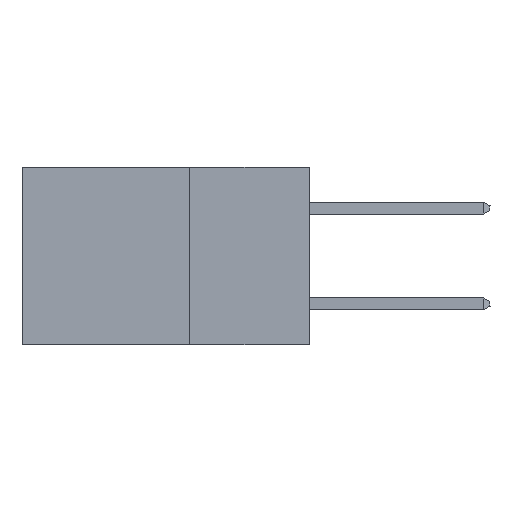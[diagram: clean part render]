
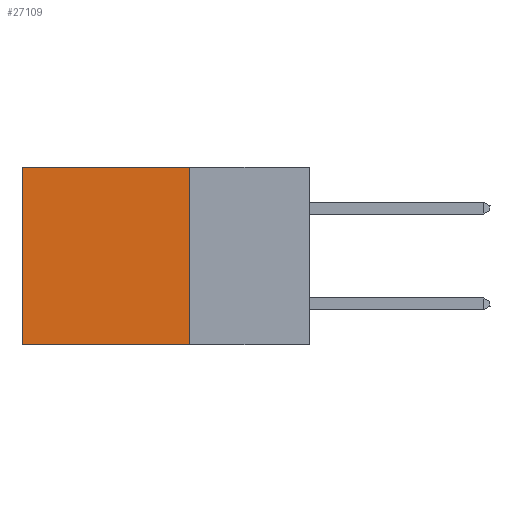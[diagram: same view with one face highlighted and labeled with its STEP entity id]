
A CAD part, left-side view. The second image highlights one B-rep face of the part: STEP entity #27109.
In plain terms, the highlighted planar face has unit normal (-1, 0, 0).
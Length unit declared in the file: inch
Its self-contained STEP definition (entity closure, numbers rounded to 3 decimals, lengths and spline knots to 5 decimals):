
#1278 = LINE ( 'NONE', #23569, #31314 ) ;
#2040 = ORIENTED_EDGE ( 'NONE', *, *, #3856, .F. ) ;
#3856 = EDGE_CURVE ( 'NONE', #38077, #13913, #1278, .T. ) ;
#4476 = ORIENTED_EDGE ( 'NONE', *, *, #10591, .F. ) ;
#5606 = ORIENTED_EDGE ( 'NONE', *, *, #35318, .T. ) ;
#9138 = VERTEX_POINT ( 'NONE', #19583 ) ;
#10522 = DIRECTION ( 'NONE',  ( 0., 0., -1. ) ) ;
#10548 = VECTOR ( 'NONE', #14507, 39.37008 ) ;
#10591 = EDGE_CURVE ( 'NONE', #13913, #19894, #17721, .T. ) ;
#12352 = AXIS2_PLACEMENT_3D ( 'NONE', #17239, #23555, #13992 ) ;
#13142 = CARTESIAN_POINT ( 'NONE',  ( 0.2875, 0.25, 0. ) ) ;
#13913 = VERTEX_POINT ( 'NONE', #36959 ) ;
#13992 = DIRECTION ( 'NONE',  ( 0., 0., -1. ) ) ;
#14507 = DIRECTION ( 'NONE',  ( 0., 1., 0. ) ) ;
#14520 = CARTESIAN_POINT ( 'NONE',  ( 0.2875, 0.6, 0. ) ) ;
#14729 = FACE_OUTER_BOUND ( 'NONE', #18526, .T. ) ;
#15652 = ORIENTED_EDGE ( 'NONE', *, *, #29291, .T. ) ;
#17239 = CARTESIAN_POINT ( 'NONE',  ( 0.2875, 0.25, 0. ) ) ;
#17721 = LINE ( 'NONE', #36675, #35751 ) ;
#18208 = LINE ( 'NONE', #14520, #34228 ) ;
#18526 = EDGE_LOOP ( 'NONE', ( #15652, #4476, #2040, #5606 ) ) ;
#19583 = CARTESIAN_POINT ( 'NONE',  ( 0.2875, 0.6, 0. ) ) ;
#19894 = VERTEX_POINT ( 'NONE', #22205 ) ;
#22205 = CARTESIAN_POINT ( 'NONE',  ( 0.2875, 0.6, -0.37 ) ) ;
#23555 = DIRECTION ( 'NONE',  ( 1., 0., 0. ) ) ;
#23569 = CARTESIAN_POINT ( 'NONE',  ( 0.2875, 0.25, 0. ) ) ;
#27109 = ADVANCED_FACE ( 'NONE', ( #14729 ), #39191, .F. ) ;
#29291 = EDGE_CURVE ( 'NONE', #9138, #19894, #18208, .T. ) ;
#31013 = CARTESIAN_POINT ( 'NONE',  ( 0.2875, 0.25, 0. ) ) ;
#31314 = VECTOR ( 'NONE', #10522, 39.37008 ) ;
#33724 = DIRECTION ( 'NONE',  ( 0., 1., 0. ) ) ;
#34228 = VECTOR ( 'NONE', #40128, 39.37008 ) ;
#34613 = LINE ( 'NONE', #31013, #10548 ) ;
#35318 = EDGE_CURVE ( 'NONE', #38077, #9138, #34613, .T. ) ;
#35751 = VECTOR ( 'NONE', #33724, 39.37008 ) ;
#36675 = CARTESIAN_POINT ( 'NONE',  ( 0.2875, 0.25, -0.37 ) ) ;
#36959 = CARTESIAN_POINT ( 'NONE',  ( 0.2875, 0.25, -0.37 ) ) ;
#38077 = VERTEX_POINT ( 'NONE', #13142 ) ;
#39191 = PLANE ( 'NONE',  #12352 ) ;
#40128 = DIRECTION ( 'NONE',  ( 0., 0., -1. ) ) ;
